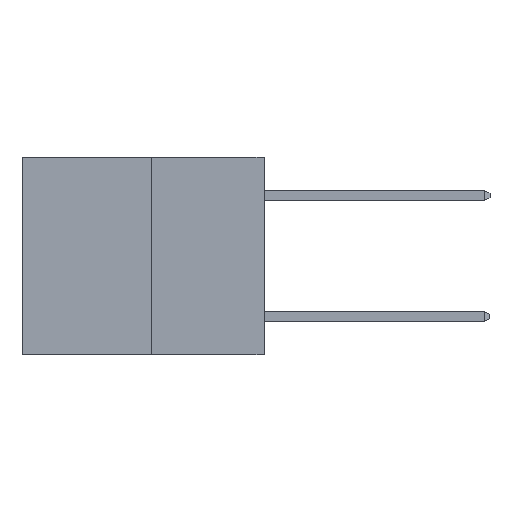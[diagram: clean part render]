
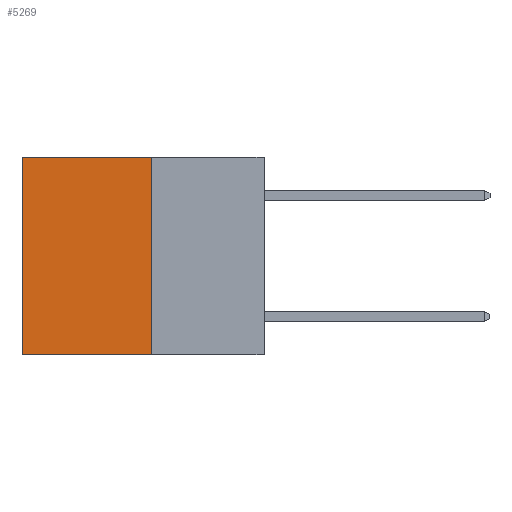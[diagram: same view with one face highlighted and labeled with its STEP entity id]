
A CAD part, left-side view. The second image highlights one B-rep face of the part: STEP entity #5269.
In plain terms, the highlighted planar face has unit normal (-1, 0, 0).
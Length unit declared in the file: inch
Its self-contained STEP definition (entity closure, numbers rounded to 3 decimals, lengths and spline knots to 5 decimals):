
#268 = VECTOR ( 'NONE', #1984, 39.37008 ) ;
#369 = LINE ( 'NONE', #8991, #11606 ) ;
#937 = DIRECTION ( 'NONE',  ( 0., 1., 0. ) ) ;
#1789 = CARTESIAN_POINT ( 'NONE',  ( 0.3165, 0.28, -0.49 ) ) ;
#1825 = DIRECTION ( 'NONE',  ( 0., 0., -1. ) ) ;
#1984 = DIRECTION ( 'NONE',  ( 0., 1., 0. ) ) ;
#2429 = DIRECTION ( 'NONE',  ( 0., 0., -1. ) ) ;
#3150 = CARTESIAN_POINT ( 'NONE',  ( 0.3165, 0.6, 0. ) ) ;
#3247 = VECTOR ( 'NONE', #1825, 39.37008 ) ;
#4464 = EDGE_CURVE ( 'NONE', #7368, #8389, #13846, .T. ) ;
#5090 = ORIENTED_EDGE ( 'NONE', *, *, #4464, .T. ) ;
#5269 = ADVANCED_FACE ( 'NONE', ( #15353 ), #13288, .F. ) ;
#5387 = EDGE_CURVE ( 'NONE', #14885, #9881, #10266, .T. ) ;
#6169 = ORIENTED_EDGE ( 'NONE', *, *, #16000, .F. ) ;
#6925 = ORIENTED_EDGE ( 'NONE', *, *, #9817, .T. ) ;
#7368 = VERTEX_POINT ( 'NONE', #12003 ) ;
#7740 = VECTOR ( 'NONE', #937, 39.37008 ) ;
#8389 = VERTEX_POINT ( 'NONE', #3150 ) ;
#8991 = CARTESIAN_POINT ( 'NONE',  ( 0.3165, 0.28, -0.49 ) ) ;
#9504 = DIRECTION ( 'NONE',  ( 1., 0., 0. ) ) ;
#9817 = EDGE_CURVE ( 'NONE', #8389, #9881, #10118, .T. ) ;
#9881 = VERTEX_POINT ( 'NONE', #10558 ) ;
#10118 = LINE ( 'NONE', #14175, #3247 ) ;
#10266 = LINE ( 'NONE', #14629, #7740 ) ;
#10558 = CARTESIAN_POINT ( 'NONE',  ( 0.3165, 0.6, -0.49 ) ) ;
#10633 = CARTESIAN_POINT ( 'NONE',  ( 0.3165, 0.28, -0.49 ) ) ;
#10803 = DIRECTION ( 'NONE',  ( 0., 0., -1. ) ) ;
#11606 = VECTOR ( 'NONE', #2429, 39.37008 ) ;
#11992 = CARTESIAN_POINT ( 'NONE',  ( 0.3165, 0.28, 0. ) ) ;
#12003 = CARTESIAN_POINT ( 'NONE',  ( 0.3165, 0.28, 0. ) ) ;
#12706 = AXIS2_PLACEMENT_3D ( 'NONE', #10633, #9504, #10803 ) ;
#13288 = PLANE ( 'NONE',  #12706 ) ;
#13810 = ORIENTED_EDGE ( 'NONE', *, *, #5387, .F. ) ;
#13846 = LINE ( 'NONE', #11992, #268 ) ;
#14175 = CARTESIAN_POINT ( 'NONE',  ( 0.3165, 0.6, -0.49 ) ) ;
#14629 = CARTESIAN_POINT ( 'NONE',  ( 0.3165, 0.28, -0.49 ) ) ;
#14885 = VERTEX_POINT ( 'NONE', #1789 ) ;
#15353 = FACE_OUTER_BOUND ( 'NONE', #15578, .T. ) ;
#15578 = EDGE_LOOP ( 'NONE', ( #6925, #13810, #6169, #5090 ) ) ;
#16000 = EDGE_CURVE ( 'NONE', #7368, #14885, #369, .T. ) ;
